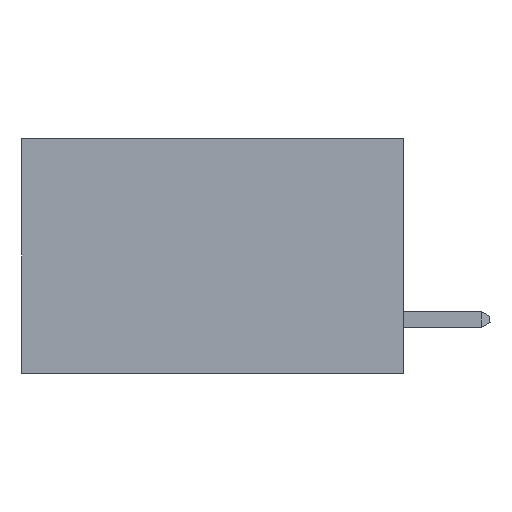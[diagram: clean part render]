
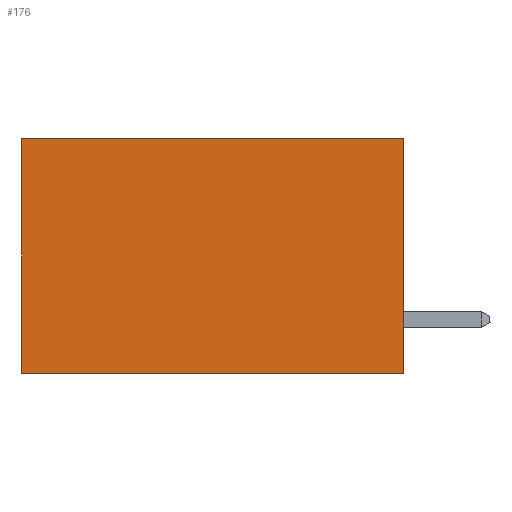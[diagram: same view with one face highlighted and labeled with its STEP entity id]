
A CAD part, left-side view. The second image highlights one B-rep face of the part: STEP entity #176.
In plain terms, the highlighted planar face has unit normal (-1, 0, 0).
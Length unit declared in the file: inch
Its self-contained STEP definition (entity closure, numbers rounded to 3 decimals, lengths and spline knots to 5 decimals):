
#149 = AXIS2_PLACEMENT_3D ( 'NONE', #14368, #8309, #1277 ) ;
#176 = ADVANCED_FACE ( 'NONE', ( #31107 ), #38116, .F. ) ;
#730 = ORIENTED_EDGE ( 'NONE', *, *, #3969, .F. ) ;
#740 = LINE ( 'NONE', #17738, #18694 ) ;
#884 = ORIENTED_EDGE ( 'NONE', *, *, #33950, .T. ) ;
#1055 = DIRECTION ( 'NONE',  ( 0., 0., -1. ) ) ;
#1277 = DIRECTION ( 'NONE',  ( 0., 0., -1. ) ) ;
#2376 = DIRECTION ( 'NONE',  ( 0., 1., 0. ) ) ;
#2835 = ORIENTED_EDGE ( 'NONE', *, *, #23505, .T. ) ;
#3478 = LINE ( 'NONE', #16972, #43594 ) ;
#3969 = EDGE_CURVE ( 'NONE', #37051, #37627, #740, .T. ) ;
#8309 = DIRECTION ( 'NONE',  ( 1., 0., 0. ) ) ;
#9159 = EDGE_CURVE ( 'NONE', #37627, #16062, #24708, .T. ) ;
#12435 = CARTESIAN_POINT ( 'NONE',  ( 0.2875, 0., -0.37 ) ) ;
#12943 = CARTESIAN_POINT ( 'NONE',  ( 0.2875, 0., 0. ) ) ;
#14368 = CARTESIAN_POINT ( 'NONE',  ( 0.2875, 0., 0. ) ) ;
#15801 = DIRECTION ( 'NONE',  ( 0., 1., 0. ) ) ;
#16062 = VERTEX_POINT ( 'NONE', #36315 ) ;
#16972 = CARTESIAN_POINT ( 'NONE',  ( 0.2875, 0., 0. ) ) ;
#17738 = CARTESIAN_POINT ( 'NONE',  ( 0.2875, 0., 0. ) ) ;
#18694 = VECTOR ( 'NONE', #1055, 39.37008 ) ;
#22094 = VERTEX_POINT ( 'NONE', #32705 ) ;
#22657 = CARTESIAN_POINT ( 'NONE',  ( 0.2875, 0., -0.37 ) ) ;
#23505 = EDGE_CURVE ( 'NONE', #37051, #22094, #3478, .T. ) ;
#24708 = LINE ( 'NONE', #12435, #31519 ) ;
#25167 = DIRECTION ( 'NONE',  ( 0., 0., -1. ) ) ;
#31107 = FACE_OUTER_BOUND ( 'NONE', #35614, .T. ) ;
#31519 = VECTOR ( 'NONE', #15801, 39.37008 ) ;
#32705 = CARTESIAN_POINT ( 'NONE',  ( 0.2875, 0.6, 0. ) ) ;
#33950 = EDGE_CURVE ( 'NONE', #22094, #16062, #41175, .T. ) ;
#35614 = EDGE_LOOP ( 'NONE', ( #884, #42494, #730, #2835 ) ) ;
#35912 = VECTOR ( 'NONE', #25167, 39.37008 ) ;
#36315 = CARTESIAN_POINT ( 'NONE',  ( 0.2875, 0.6, -0.37 ) ) ;
#37051 = VERTEX_POINT ( 'NONE', #12943 ) ;
#37627 = VERTEX_POINT ( 'NONE', #22657 ) ;
#38116 = PLANE ( 'NONE',  #149 ) ;
#38408 = CARTESIAN_POINT ( 'NONE',  ( 0.2875, 0.6, 0. ) ) ;
#41175 = LINE ( 'NONE', #38408, #35912 ) ;
#42494 = ORIENTED_EDGE ( 'NONE', *, *, #9159, .F. ) ;
#43594 = VECTOR ( 'NONE', #2376, 39.37008 ) ;
